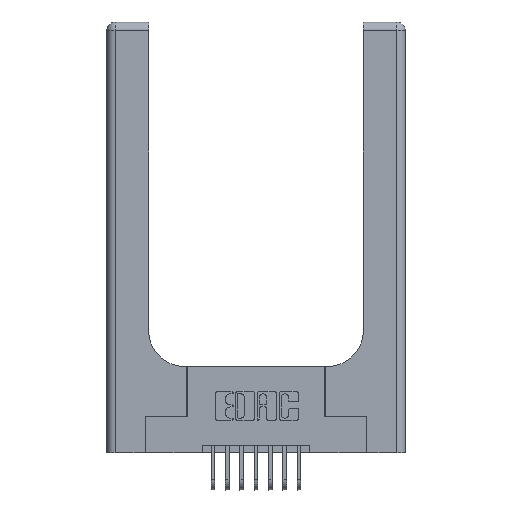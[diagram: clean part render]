
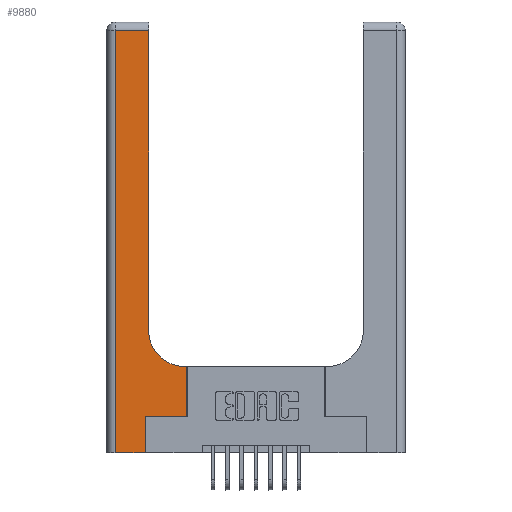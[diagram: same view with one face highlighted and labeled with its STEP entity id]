
A CAD part, top view. The second image highlights one B-rep face of the part: STEP entity #9880.
In plain terms, the highlighted planar face has unit normal (0, 0, 1).
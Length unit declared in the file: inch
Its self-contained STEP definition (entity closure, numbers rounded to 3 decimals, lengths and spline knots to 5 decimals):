
#228 = LINE ( 'NONE', #997, #9997 ) ;
#419 = PLANE ( 'NONE',  #4649 ) ;
#873 = ORIENTED_EDGE ( 'NONE', *, *, #4897, .T. ) ;
#997 = CARTESIAN_POINT ( 'NONE',  ( 0.2915, 0.6, 0.37 ) ) ;
#1028 = VECTOR ( 'NONE', #10123, 39.37008 ) ;
#1036 = CARTESIAN_POINT ( 'NONE',  ( 0.5415, 0.85, 0.37 ) ) ;
#1187 = EDGE_CURVE ( 'NONE', #13720, #8986, #9337, .T. ) ;
#1417 = CARTESIAN_POINT ( 'NONE',  ( 0.06, 2.94, 0.37 ) ) ;
#1641 = CARTESIAN_POINT ( 'NONE',  ( 0.2915, 0.85, 0.37 ) ) ;
#1694 = DIRECTION ( 'NONE',  ( 0., 1., 0. ) ) ;
#1930 = ORIENTED_EDGE ( 'NONE', *, *, #8702, .T. ) ;
#2185 = CARTESIAN_POINT ( 'NONE',  ( 0.269, 0., 0.37 ) ) ;
#2199 = VECTOR ( 'NONE', #12949, 39.37008 ) ;
#2205 = DIRECTION ( 'NONE',  ( 1., 0., 0. ) ) ;
#2294 = VERTEX_POINT ( 'NONE', #6496 ) ;
#2358 = CARTESIAN_POINT ( 'NONE',  ( 0., 2.94, 0.37 ) ) ;
#2436 = VERTEX_POINT ( 'NONE', #2185 ) ;
#2727 = ORIENTED_EDGE ( 'NONE', *, *, #13000, .T. ) ;
#2786 = DIRECTION ( 'NONE',  ( 0., 0., -1. ) ) ;
#2858 = CARTESIAN_POINT ( 'NONE',  ( 0.5585, 0.25, 0.37 ) ) ;
#3047 = CARTESIAN_POINT ( 'NONE',  ( 0.5585, 0.6, 0.37 ) ) ;
#3359 = ORIENTED_EDGE ( 'NONE', *, *, #11182, .T. ) ;
#3439 = VECTOR ( 'NONE', #8004, 39.37008 ) ;
#3448 = EDGE_CURVE ( 'NONE', #2294, #6676, #12392, .T. ) ;
#3850 = DIRECTION ( 'NONE',  ( 1., 0., 0. ) ) ;
#3984 = EDGE_CURVE ( 'NONE', #6676, #14569, #15114, .T. ) ;
#4061 = LINE ( 'NONE', #2858, #9948 ) ;
#4134 = LINE ( 'NONE', #4255, #1028 ) ;
#4255 = CARTESIAN_POINT ( 'NONE',  ( 0.269, 0., 0.37 ) ) ;
#4649 = AXIS2_PLACEMENT_3D ( 'NONE', #9821, #2786, #11001 ) ;
#4692 = FACE_OUTER_BOUND ( 'NONE', #14804, .T. ) ;
#4897 = EDGE_CURVE ( 'NONE', #13961, #5012, #4061, .T. ) ;
#5012 = VERTEX_POINT ( 'NONE', #3047 ) ;
#5312 = CARTESIAN_POINT ( 'NONE',  ( 0.2915, 2.94, 0.37 ) ) ;
#5744 = ORIENTED_EDGE ( 'NONE', *, *, #3984, .T. ) ;
#5996 = EDGE_CURVE ( 'NONE', #14569, #13720, #8440, .T. ) ;
#6449 = VECTOR ( 'NONE', #11773, 39.37008 ) ;
#6496 = CARTESIAN_POINT ( 'NONE',  ( 0.5415, 0.6, 0.37 ) ) ;
#6676 = VERTEX_POINT ( 'NONE', #1641 ) ;
#6681 = AXIS2_PLACEMENT_3D ( 'NONE', #1036, #9257, #2205 ) ;
#6820 = ORIENTED_EDGE ( 'NONE', *, *, #5996, .T. ) ;
#7094 = ORIENTED_EDGE ( 'NONE', *, *, #3448, .T. ) ;
#7206 = ORIENTED_EDGE ( 'NONE', *, *, #1187, .T. ) ;
#7271 = LINE ( 'NONE', #13262, #10039 ) ;
#8004 = DIRECTION ( 'NONE',  ( 0., -1., 0. ) ) ;
#8037 = CARTESIAN_POINT ( 'NONE',  ( 0.06, 3., 0.37 ) ) ;
#8440 = LINE ( 'NONE', #2358, #2199 ) ;
#8486 = VERTEX_POINT ( 'NONE', #10430 ) ;
#8702 = EDGE_CURVE ( 'NONE', #8486, #13961, #7271, .T. ) ;
#8986 = VERTEX_POINT ( 'NONE', #13766 ) ;
#9207 = DIRECTION ( 'NONE',  ( -1., 0., 0. ) ) ;
#9257 = DIRECTION ( 'NONE',  ( 0., 0., -1. ) ) ;
#9337 = LINE ( 'NONE', #8037, #3439 ) ;
#9821 = CARTESIAN_POINT ( 'NONE',  ( 0., 3., 0.37 ) ) ;
#9880 = ADVANCED_FACE ( 'NONE', ( #4692 ), #419, .F. ) ;
#9948 = VECTOR ( 'NONE', #1694, 39.37008 ) ;
#9997 = VECTOR ( 'NONE', #9207, 39.37008 ) ;
#10039 = VECTOR ( 'NONE', #3850, 39.37008 ) ;
#10123 = DIRECTION ( 'NONE',  ( 0., 1., 0. ) ) ;
#10430 = CARTESIAN_POINT ( 'NONE',  ( 0.269, 0.25, 0.37 ) ) ;
#10584 = CARTESIAN_POINT ( 'NONE',  ( 0., 0., 0.37 ) ) ;
#11001 = DIRECTION ( 'NONE',  ( -1., 0., 0. ) ) ;
#11182 = EDGE_CURVE ( 'NONE', #2436, #8486, #4134, .T. ) ;
#11434 = CARTESIAN_POINT ( 'NONE',  ( 0.2915, 3., 0.37 ) ) ;
#11773 = DIRECTION ( 'NONE',  ( 1., 0., 0. ) ) ;
#12349 = LINE ( 'NONE', #10584, #6449 ) ;
#12392 = CIRCLE ( 'NONE', #6681, 0.25 ) ;
#12620 = DIRECTION ( 'NONE',  ( 0., 1., 0. ) ) ;
#12949 = DIRECTION ( 'NONE',  ( -1., 0., 0. ) ) ;
#13000 = EDGE_CURVE ( 'NONE', #5012, #2294, #228, .T. ) ;
#13262 = CARTESIAN_POINT ( 'NONE',  ( 0.269, 0.25, 0.37 ) ) ;
#13492 = CARTESIAN_POINT ( 'NONE',  ( 0.5585, 0.25, 0.37 ) ) ;
#13720 = VERTEX_POINT ( 'NONE', #1417 ) ;
#13766 = CARTESIAN_POINT ( 'NONE',  ( 0.06, 0., 0.37 ) ) ;
#13961 = VERTEX_POINT ( 'NONE', #13492 ) ;
#14320 = EDGE_CURVE ( 'NONE', #8986, #2436, #12349, .T. ) ;
#14569 = VERTEX_POINT ( 'NONE', #5312 ) ;
#14759 = VECTOR ( 'NONE', #12620, 39.37008 ) ;
#14804 = EDGE_LOOP ( 'NONE', ( #5744, #6820, #7206, #14818, #3359, #1930, #873, #2727, #7094 ) ) ;
#14818 = ORIENTED_EDGE ( 'NONE', *, *, #14320, .T. ) ;
#15114 = LINE ( 'NONE', #11434, #14759 ) ;
